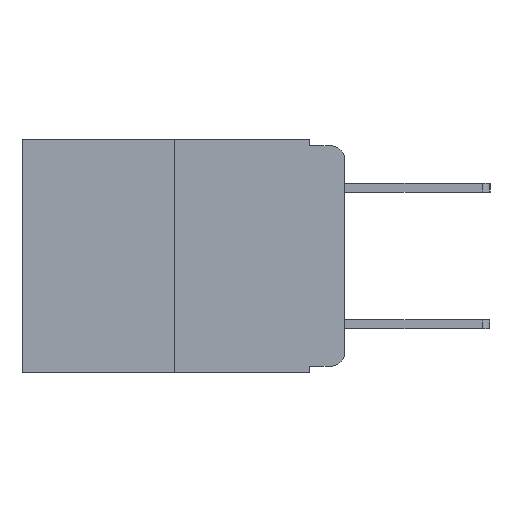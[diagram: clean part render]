
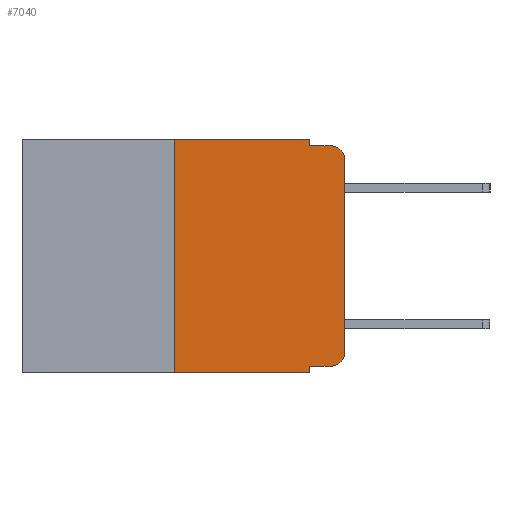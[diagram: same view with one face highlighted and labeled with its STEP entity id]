
A CAD part, left-side view. The second image highlights one B-rep face of the part: STEP entity #7040.
In plain terms, the highlighted planar face has unit normal (-1, 0, 0).
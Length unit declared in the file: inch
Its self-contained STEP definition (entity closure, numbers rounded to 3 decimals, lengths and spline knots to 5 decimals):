
#125 = DIRECTION ( 'NONE',  ( -1., 0., 0. ) ) ;
#172 = LINE ( 'NONE', #11843, #15281 ) ;
#250 = CARTESIAN_POINT ( 'NONE',  ( 0., 0.051, 0. ) ) ;
#361 = DIRECTION ( 'NONE',  ( 0., -1., 0. ) ) ;
#399 = CARTESIAN_POINT ( 'NONE',  ( 0., 0.051, -0.333 ) ) ;
#620 = CARTESIAN_POINT ( 'NONE',  ( 0., 0.051, -0.01 ) ) ;
#822 = CARTESIAN_POINT ( 'NONE',  ( 0., 0.051, -0.333 ) ) ;
#1009 = VERTEX_POINT ( 'NONE', #14767 ) ;
#1030 = ORIENTED_EDGE ( 'NONE', *, *, #3380, .F. ) ;
#1335 = CARTESIAN_POINT ( 'NONE',  ( 0., 0., -0.03 ) ) ;
#1358 = DIRECTION ( 'NONE',  ( 0., -1., 0. ) ) ;
#1401 = LINE ( 'NONE', #620, #7773 ) ;
#1515 = CARTESIAN_POINT ( 'NONE',  ( 0., 0.473, -0.343 ) ) ;
#1537 = VERTEX_POINT ( 'NONE', #14253 ) ;
#1621 = EDGE_CURVE ( 'NONE', #1009, #10660, #2584, .T. ) ;
#1623 = EDGE_CURVE ( 'NONE', #10660, #1537, #12965, .T. ) ;
#1645 = EDGE_CURVE ( 'NONE', #10280, #1537, #1401, .T. ) ;
#1669 = EDGE_CURVE ( 'NONE', #14579, #10280, #7395, .T. ) ;
#1698 = CARTESIAN_POINT ( 'NONE',  ( 0., 0.051, -0.343 ) ) ;
#1867 = DIRECTION ( 'NONE',  ( 0., -1., 0. ) ) ;
#2188 = AXIS2_PLACEMENT_3D ( 'NONE', #5504, #4190, #8061 ) ;
#2192 = LINE ( 'NONE', #1515, #5613 ) ;
#2292 = EDGE_CURVE ( 'NONE', #7597, #13856, #13927, .T. ) ;
#2336 = EDGE_LOOP ( 'NONE', ( #2396, #6184, #15326, #9848, #12808, #13141, #3967, #1030, #4393, #10929 ) ) ;
#2396 = ORIENTED_EDGE ( 'NONE', *, *, #1621, .T. ) ;
#2399 = DIRECTION ( 'NONE',  ( 0., 0., 1. ) ) ;
#2492 = DIRECTION ( 'NONE',  ( 0., 0., -1. ) ) ;
#2584 = LINE ( 'NONE', #6489, #8944 ) ;
#2764 = DIRECTION ( 'NONE',  ( 0., -1., 0. ) ) ;
#3380 = EDGE_CURVE ( 'NONE', #14891, #7060, #172, .T. ) ;
#3523 = EDGE_CURVE ( 'NONE', #14891, #11645, #15447, .T. ) ;
#3592 = EDGE_CURVE ( 'NONE', #11645, #1009, #13411, .T. ) ;
#3593 = FACE_OUTER_BOUND ( 'NONE', #2336, .T. ) ;
#3967 = ORIENTED_EDGE ( 'NONE', *, *, #15309, .T. ) ;
#4093 = DIRECTION ( 'NONE',  ( 0., 0., -1. ) ) ;
#4190 = DIRECTION ( 'NONE',  ( 1., 0., 0. ) ) ;
#4393 = ORIENTED_EDGE ( 'NONE', *, *, #3523, .T. ) ;
#4406 = DIRECTION ( 'NONE',  ( 0., 0., 1. ) ) ;
#4425 = CARTESIAN_POINT ( 'NONE',  ( 0., 0.473, 0. ) ) ;
#4558 = AXIS2_PLACEMENT_3D ( 'NONE', #7750, #125, #4093 ) ;
#5504 = CARTESIAN_POINT ( 'NONE',  ( 0., 0.473, 0. ) ) ;
#5613 = VECTOR ( 'NONE', #2764, 39.37008 ) ;
#6124 = DIRECTION ( 'NONE',  ( 0., 0., -1. ) ) ;
#6173 = AXIS2_PLACEMENT_3D ( 'NONE', #9731, #9877, #2492 ) ;
#6184 = ORIENTED_EDGE ( 'NONE', *, *, #1623, .T. ) ;
#6331 = VECTOR ( 'NONE', #361, 39.37008 ) ;
#6489 = CARTESIAN_POINT ( 'NONE',  ( 0., 0., 0. ) ) ;
#7002 = VECTOR ( 'NONE', #15400, 39.37008 ) ;
#7040 = ADVANCED_FACE ( 'NONE', ( #3593 ), #14738, .F. ) ;
#7060 = VERTEX_POINT ( 'NONE', #1698 ) ;
#7266 = CARTESIAN_POINT ( 'NONE',  ( 0., 0.051, -0.01 ) ) ;
#7384 = LINE ( 'NONE', #4425, #10208 ) ;
#7395 = LINE ( 'NONE', #250, #7002 ) ;
#7505 = CARTESIAN_POINT ( 'NONE',  ( 0., 0.02, -0.333 ) ) ;
#7597 = VERTEX_POINT ( 'NONE', #10320 ) ;
#7750 = CARTESIAN_POINT ( 'NONE',  ( 0., 0.02, -0.03 ) ) ;
#7773 = VECTOR ( 'NONE', #1358, 39.37008 ) ;
#8061 = DIRECTION ( 'NONE',  ( 0., 0., -1. ) ) ;
#8406 = CARTESIAN_POINT ( 'NONE',  ( 0., 0.051, 0. ) ) ;
#8944 = VECTOR ( 'NONE', #2399, 39.37008 ) ;
#9731 = CARTESIAN_POINT ( 'NONE',  ( 0., 0.02, -0.313 ) ) ;
#9848 = ORIENTED_EDGE ( 'NONE', *, *, #1669, .F. ) ;
#9877 = DIRECTION ( 'NONE',  ( -1., 0., 0. ) ) ;
#10208 = VECTOR ( 'NONE', #1867, 39.37008 ) ;
#10280 = VERTEX_POINT ( 'NONE', #7266 ) ;
#10320 = CARTESIAN_POINT ( 'NONE',  ( 0., 0.25, -0.343 ) ) ;
#10660 = VERTEX_POINT ( 'NONE', #1335 ) ;
#10929 = ORIENTED_EDGE ( 'NONE', *, *, #3592, .T. ) ;
#11645 = VERTEX_POINT ( 'NONE', #7505 ) ;
#11843 = CARTESIAN_POINT ( 'NONE',  ( 0., 0.051, 0. ) ) ;
#12483 = CARTESIAN_POINT ( 'NONE',  ( 0., 0.25, 0. ) ) ;
#12808 = ORIENTED_EDGE ( 'NONE', *, *, #14476, .F. ) ;
#12965 = CIRCLE ( 'NONE', #4558, 0.02 ) ;
#13141 = ORIENTED_EDGE ( 'NONE', *, *, #2292, .F. ) ;
#13411 = CIRCLE ( 'NONE', #6173, 0.02 ) ;
#13596 = VECTOR ( 'NONE', #4406, 39.37008 ) ;
#13856 = VERTEX_POINT ( 'NONE', #15156 ) ;
#13927 = LINE ( 'NONE', #12483, #13596 ) ;
#14253 = CARTESIAN_POINT ( 'NONE',  ( 0., 0.02, -0.01 ) ) ;
#14476 = EDGE_CURVE ( 'NONE', #13856, #14579, #7384, .T. ) ;
#14579 = VERTEX_POINT ( 'NONE', #8406 ) ;
#14738 = PLANE ( 'NONE',  #2188 ) ;
#14767 = CARTESIAN_POINT ( 'NONE',  ( 0., 0., -0.313 ) ) ;
#14891 = VERTEX_POINT ( 'NONE', #822 ) ;
#15156 = CARTESIAN_POINT ( 'NONE',  ( 0., 0.25, 0. ) ) ;
#15281 = VECTOR ( 'NONE', #6124, 39.37008 ) ;
#15309 = EDGE_CURVE ( 'NONE', #7597, #7060, #2192, .T. ) ;
#15326 = ORIENTED_EDGE ( 'NONE', *, *, #1645, .F. ) ;
#15400 = DIRECTION ( 'NONE',  ( 0., 0., -1. ) ) ;
#15447 = LINE ( 'NONE', #399, #6331 ) ;
